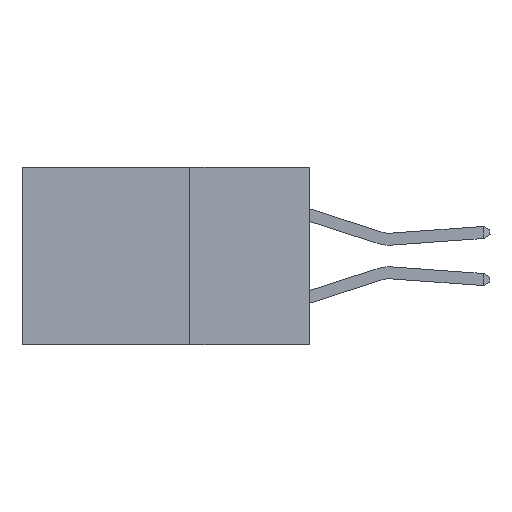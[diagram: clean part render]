
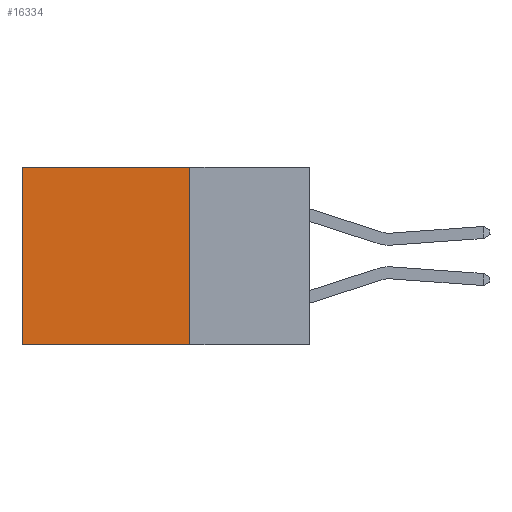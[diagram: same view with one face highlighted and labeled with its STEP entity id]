
A CAD part, left-side view. The second image highlights one B-rep face of the part: STEP entity #16334.
In plain terms, the highlighted planar face has unit normal (-1, 0, 0).
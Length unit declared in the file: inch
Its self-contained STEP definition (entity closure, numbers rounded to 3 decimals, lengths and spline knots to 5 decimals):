
#98 = VERTEX_POINT ( 'NONE', #23346 ) ;
#747 = DIRECTION ( 'NONE',  ( 0., 0., -1. ) ) ;
#1355 = VECTOR ( 'NONE', #21668, 39.37008 ) ;
#2266 = ORIENTED_EDGE ( 'NONE', *, *, #4338, .T. ) ;
#2298 = VECTOR ( 'NONE', #747, 39.37008 ) ;
#2877 = CARTESIAN_POINT ( 'NONE',  ( 0.2615, 0.25, 0. ) ) ;
#2928 = CARTESIAN_POINT ( 'NONE',  ( 0.2615, 0.25, -0.37 ) ) ;
#4338 = EDGE_CURVE ( 'NONE', #22921, #19553, #20676, .T. ) ;
#4373 = ORIENTED_EDGE ( 'NONE', *, *, #26008, .F. ) ;
#4470 = AXIS2_PLACEMENT_3D ( 'NONE', #15124, #21369, #26035 ) ;
#5849 = ORIENTED_EDGE ( 'NONE', *, *, #24138, .F. ) ;
#5865 = CARTESIAN_POINT ( 'NONE',  ( 0.2615, 0.6, 0. ) ) ;
#6235 = ORIENTED_EDGE ( 'NONE', *, *, #13405, .T. ) ;
#6650 = VERTEX_POINT ( 'NONE', #20346 ) ;
#8149 = LINE ( 'NONE', #14332, #23560 ) ;
#9116 = CARTESIAN_POINT ( 'NONE',  ( 0.2615, 0.6, -0.37 ) ) ;
#9121 = DIRECTION ( 'NONE',  ( 0., 1., 0. ) ) ;
#12579 = DIRECTION ( 'NONE',  ( 0., 0., -1. ) ) ;
#13405 = EDGE_CURVE ( 'NONE', #6650, #22921, #21258, .T. ) ;
#13699 = VECTOR ( 'NONE', #9121, 39.37008 ) ;
#14332 = CARTESIAN_POINT ( 'NONE',  ( 0.2615, 0.25, -0.37 ) ) ;
#15124 = CARTESIAN_POINT ( 'NONE',  ( 0.2615, 0.25, -0.37 ) ) ;
#16334 = ADVANCED_FACE ( 'NONE', ( #17171 ), #25481, .F. ) ;
#17171 = FACE_OUTER_BOUND ( 'NONE', #24633, .T. ) ;
#19553 = VERTEX_POINT ( 'NONE', #22117 ) ;
#19682 = LINE ( 'NONE', #2928, #13699 ) ;
#20346 = CARTESIAN_POINT ( 'NONE',  ( 0.2615, 0.25, 0. ) ) ;
#20676 = LINE ( 'NONE', #9116, #2298 ) ;
#21258 = LINE ( 'NONE', #2877, #1355 ) ;
#21369 = DIRECTION ( 'NONE',  ( 1., 0., 0. ) ) ;
#21668 = DIRECTION ( 'NONE',  ( 0., 1., 0. ) ) ;
#22117 = CARTESIAN_POINT ( 'NONE',  ( 0.2615, 0.6, -0.37 ) ) ;
#22921 = VERTEX_POINT ( 'NONE', #5865 ) ;
#23346 = CARTESIAN_POINT ( 'NONE',  ( 0.2615, 0.25, -0.37 ) ) ;
#23560 = VECTOR ( 'NONE', #12579, 39.37008 ) ;
#24138 = EDGE_CURVE ( 'NONE', #98, #19553, #19682, .T. ) ;
#24633 = EDGE_LOOP ( 'NONE', ( #2266, #5849, #4373, #6235 ) ) ;
#25481 = PLANE ( 'NONE',  #4470 ) ;
#26008 = EDGE_CURVE ( 'NONE', #6650, #98, #8149, .T. ) ;
#26035 = DIRECTION ( 'NONE',  ( 0., 0., -1. ) ) ;
